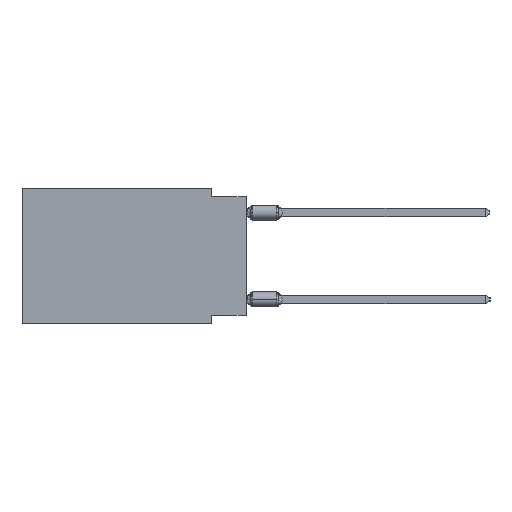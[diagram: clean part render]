
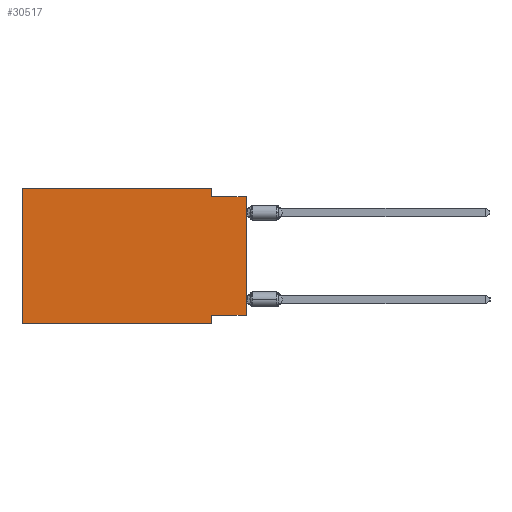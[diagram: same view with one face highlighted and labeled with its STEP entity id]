
A CAD part, left-side view. The second image highlights one B-rep face of the part: STEP entity #30517.
In plain terms, the highlighted planar face has unit normal (-1, 0, 0).
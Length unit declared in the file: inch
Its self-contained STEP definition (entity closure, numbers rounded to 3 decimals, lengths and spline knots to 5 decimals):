
#632 = EDGE_CURVE ( 'NONE', #4360, #34509, #14622, .T. ) ;
#2275 = LINE ( 'NONE', #8346, #12410 ) ;
#2887 = EDGE_CURVE ( 'NONE', #23067, #9914, #10295, .T. ) ;
#2966 = EDGE_CURVE ( 'NONE', #4360, #4737, #7069, .T. ) ;
#4220 = ORIENTED_EDGE ( 'NONE', *, *, #8666, .F. ) ;
#4360 = VERTEX_POINT ( 'NONE', #31237 ) ;
#4737 = VERTEX_POINT ( 'NONE', #21893 ) ;
#5306 = DIRECTION ( 'NONE',  ( 0., -1., 0. ) ) ;
#5806 = DIRECTION ( 'NONE',  ( 0., -1., 0. ) ) ;
#5841 = EDGE_CURVE ( 'NONE', #23067, #21357, #26086, .T. ) ;
#6226 = CARTESIAN_POINT ( 'NONE',  ( 0., 0., 0. ) ) ;
#6417 = ORIENTED_EDGE ( 'NONE', *, *, #5841, .T. ) ;
#7069 = LINE ( 'NONE', #12609, #26414 ) ;
#8316 = AXIS2_PLACEMENT_3D ( 'NONE', #34875, #16036, #32171 ) ;
#8346 = CARTESIAN_POINT ( 'NONE',  ( 0., 0., -0.025 ) ) ;
#8666 = EDGE_CURVE ( 'NONE', #11925, #34509, #2275, .T. ) ;
#8683 = ORIENTED_EDGE ( 'NONE', *, *, #30734, .F. ) ;
#8714 = ORIENTED_EDGE ( 'NONE', *, *, #32739, .F. ) ;
#9914 = VERTEX_POINT ( 'NONE', #24295 ) ;
#10295 = LINE ( 'NONE', #34684, #33275 ) ;
#11039 = EDGE_CURVE ( 'NONE', #9914, #23011, #13841, .T. ) ;
#11925 = VERTEX_POINT ( 'NONE', #32065 ) ;
#12410 = VECTOR ( 'NONE', #5306, 39.37008 ) ;
#12609 = CARTESIAN_POINT ( 'NONE',  ( 0., 0., -0.365 ) ) ;
#12968 = CARTESIAN_POINT ( 'NONE',  ( 0., 0.1, 0. ) ) ;
#13200 = ORIENTED_EDGE ( 'NONE', *, *, #2966, .F. ) ;
#13411 = LINE ( 'NONE', #32990, #17572 ) ;
#13841 = LINE ( 'NONE', #27486, #23251 ) ;
#14622 = LINE ( 'NONE', #6226, #25047 ) ;
#14758 = DIRECTION ( 'NONE',  ( 0., 0., -1. ) ) ;
#16036 = DIRECTION ( 'NONE',  ( 1., 0., 0. ) ) ;
#16777 = EDGE_LOOP ( 'NONE', ( #22551, #4220, #8714, #33659, #22146, #6417, #8683, #13200 ) ) ;
#16788 = DIRECTION ( 'NONE',  ( 0., 0., 1. ) ) ;
#17572 = VECTOR ( 'NONE', #32447, 39.37008 ) ;
#19609 = CARTESIAN_POINT ( 'NONE',  ( 0., 0.645, -0.39 ) ) ;
#20156 = CARTESIAN_POINT ( 'NONE',  ( 0., 0.1, -0.39 ) ) ;
#20906 = VECTOR ( 'NONE', #14758, 39.37008 ) ;
#21357 = VERTEX_POINT ( 'NONE', #20156 ) ;
#21893 = CARTESIAN_POINT ( 'NONE',  ( 0., 0.1, -0.365 ) ) ;
#22146 = ORIENTED_EDGE ( 'NONE', *, *, #2887, .F. ) ;
#22551 = ORIENTED_EDGE ( 'NONE', *, *, #632, .T. ) ;
#23011 = VERTEX_POINT ( 'NONE', #12968 ) ;
#23067 = VERTEX_POINT ( 'NONE', #19609 ) ;
#23251 = VECTOR ( 'NONE', #5806, 39.37008 ) ;
#23274 = CARTESIAN_POINT ( 'NONE',  ( 0., 0., -0.025 ) ) ;
#23567 = FACE_OUTER_BOUND ( 'NONE', #16777, .T. ) ;
#24295 = CARTESIAN_POINT ( 'NONE',  ( 0., 0.645, 0. ) ) ;
#25047 = VECTOR ( 'NONE', #16788, 39.37008 ) ;
#25521 = CARTESIAN_POINT ( 'NONE',  ( 0., 0.1, -0.39 ) ) ;
#25701 = LINE ( 'NONE', #25521, #20906 ) ;
#26086 = LINE ( 'NONE', #29127, #29347 ) ;
#26414 = VECTOR ( 'NONE', #28926, 39.37008 ) ;
#27486 = CARTESIAN_POINT ( 'NONE',  ( 0., 0.645, 0. ) ) ;
#28926 = DIRECTION ( 'NONE',  ( 0., 1., 0. ) ) ;
#29127 = CARTESIAN_POINT ( 'NONE',  ( 0., 0.645, -0.39 ) ) ;
#29347 = VECTOR ( 'NONE', #34347, 39.37008 ) ;
#30517 = ADVANCED_FACE ( 'NONE', ( #23567 ), #31646, .F. ) ;
#30734 = EDGE_CURVE ( 'NONE', #4737, #21357, #25701, .T. ) ;
#31237 = CARTESIAN_POINT ( 'NONE',  ( 0., 0., -0.365 ) ) ;
#31646 = PLANE ( 'NONE',  #8316 ) ;
#32065 = CARTESIAN_POINT ( 'NONE',  ( 0., 0.1, -0.025 ) ) ;
#32171 = DIRECTION ( 'NONE',  ( 0., 0., -1. ) ) ;
#32447 = DIRECTION ( 'NONE',  ( 0., 0., -1. ) ) ;
#32739 = EDGE_CURVE ( 'NONE', #23011, #11925, #13411, .T. ) ;
#32990 = CARTESIAN_POINT ( 'NONE',  ( 0., 0.1, 0. ) ) ;
#33275 = VECTOR ( 'NONE', #35029, 39.37008 ) ;
#33659 = ORIENTED_EDGE ( 'NONE', *, *, #11039, .F. ) ;
#34347 = DIRECTION ( 'NONE',  ( 0., -1., 0. ) ) ;
#34509 = VERTEX_POINT ( 'NONE', #23274 ) ;
#34684 = CARTESIAN_POINT ( 'NONE',  ( 0., 0.645, 0. ) ) ;
#34875 = CARTESIAN_POINT ( 'NONE',  ( 0., 0.645, 0. ) ) ;
#35029 = DIRECTION ( 'NONE',  ( 0., 0., 1. ) ) ;
